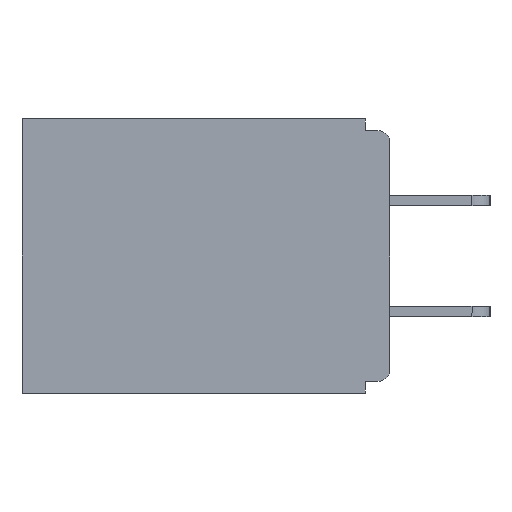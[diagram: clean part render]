
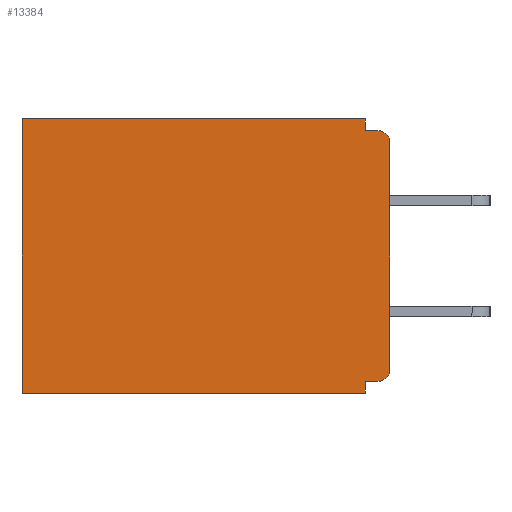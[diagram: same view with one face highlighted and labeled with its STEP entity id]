
A CAD part, left-side view. The second image highlights one B-rep face of the part: STEP entity #13384.
In plain terms, the highlighted planar face has unit normal (-1, 0, 0).
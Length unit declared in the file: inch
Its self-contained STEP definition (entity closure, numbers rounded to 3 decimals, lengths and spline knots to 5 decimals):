
#208 = DIRECTION ( 'NONE',  ( 0., 1., 0. ) ) ;
#1018 = DIRECTION ( 'NONE',  ( 0., 0., -1. ) ) ;
#1232 = CARTESIAN_POINT ( 'NONE',  ( 0.298, 0., -0.015 ) ) ;
#1733 = VECTOR ( 'NONE', #10313, 39.37008 ) ;
#1780 = ORIENTED_EDGE ( 'NONE', *, *, #7760, .T. ) ;
#2868 = EDGE_CURVE ( 'NONE', #8857, #16512, #18832, .T. ) ;
#3001 = ORIENTED_EDGE ( 'NONE', *, *, #2868, .F. ) ;
#3251 = ORIENTED_EDGE ( 'NONE', *, *, #22181, .T. ) ;
#3342 = DIRECTION ( 'NONE',  ( 0., 0., -1. ) ) ;
#3400 = EDGE_CURVE ( 'NONE', #14021, #8857, #15258, .T. ) ;
#3413 = CARTESIAN_POINT ( 'NONE',  ( 0.298, 0.015, -0.015 ) ) ;
#3525 = VECTOR ( 'NONE', #6233, 39.37008 ) ;
#3617 = ORIENTED_EDGE ( 'NONE', *, *, #11317, .F. ) ;
#3928 = EDGE_LOOP ( 'NONE', ( #3251, #20395, #15537, #11468, #1780, #3617, #3001, #13263, #16949, #18435 ) ) ;
#4013 = VERTEX_POINT ( 'NONE', #3413 ) ;
#4075 = DIRECTION ( 'NONE',  ( 0., 0., -1. ) ) ;
#4299 = AXIS2_PLACEMENT_3D ( 'NONE', #11005, #13020, #3342 ) ;
#4337 = EDGE_CURVE ( 'NONE', #23178, #23728, #9349, .T. ) ;
#4567 = EDGE_CURVE ( 'NONE', #14021, #17138, #11123, .T. ) ;
#4752 = FACE_OUTER_BOUND ( 'NONE', #3928, .T. ) ;
#5215 = DIRECTION ( 'NONE',  ( 0., -1., 0. ) ) ;
#5217 = CARTESIAN_POINT ( 'NONE',  ( 0.298, 0., -0.313 ) ) ;
#5281 = DIRECTION ( 'NONE',  ( 0., 0., -1. ) ) ;
#5298 = VECTOR ( 'NONE', #5281, 39.37008 ) ;
#5669 = CARTESIAN_POINT ( 'NONE',  ( 0.298, 0., -0.343 ) ) ;
#6160 = CARTESIAN_POINT ( 'NONE',  ( 0.298, 0.46, -0.343 ) ) ;
#6233 = DIRECTION ( 'NONE',  ( 0., 0., -1. ) ) ;
#6767 = LINE ( 'NONE', #22527, #5298 ) ;
#6958 = VECTOR ( 'NONE', #13476, 39.37008 ) ;
#7760 = EDGE_CURVE ( 'NONE', #23728, #24409, #6767, .T. ) ;
#8609 = CARTESIAN_POINT ( 'NONE',  ( 0.298, 0.46, 0. ) ) ;
#8857 = VERTEX_POINT ( 'NONE', #24695 ) ;
#9024 = LINE ( 'NONE', #20886, #12075 ) ;
#9349 = LINE ( 'NONE', #19607, #14158 ) ;
#9690 = CARTESIAN_POINT ( 'NONE',  ( 0.298, 0., 0. ) ) ;
#10313 = DIRECTION ( 'NONE',  ( 0., 1., 0. ) ) ;
#10436 = AXIS2_PLACEMENT_3D ( 'NONE', #10706, #18234, #1018 ) ;
#10706 = CARTESIAN_POINT ( 'NONE',  ( 0.298, 0.015, -0.313 ) ) ;
#10724 = LINE ( 'NONE', #9690, #24216 ) ;
#11005 = CARTESIAN_POINT ( 'NONE',  ( 0.298, 0., 0. ) ) ;
#11123 = CIRCLE ( 'NONE', #10436, 0.015 ) ;
#11317 = EDGE_CURVE ( 'NONE', #16512, #24409, #21636, .T. ) ;
#11468 = ORIENTED_EDGE ( 'NONE', *, *, #4337, .T. ) ;
#11710 = VERTEX_POINT ( 'NONE', #21645 ) ;
#11959 = EDGE_CURVE ( 'NONE', #23178, #17502, #9024, .T. ) ;
#12075 = VECTOR ( 'NONE', #13386, 39.37008 ) ;
#12385 = LINE ( 'NONE', #1232, #14745 ) ;
#12413 = CARTESIAN_POINT ( 'NONE',  ( 0.298, 0.031, 0. ) ) ;
#13020 = DIRECTION ( 'NONE',  ( 1., 0., 0. ) ) ;
#13126 = CARTESIAN_POINT ( 'NONE',  ( 0.298, 0.015, -0.328 ) ) ;
#13263 = ORIENTED_EDGE ( 'NONE', *, *, #3400, .F. ) ;
#13384 = ADVANCED_FACE ( 'NONE', ( #4752 ), #22449, .F. ) ;
#13386 = DIRECTION ( 'NONE',  ( 0., 0., -1. ) ) ;
#13476 = DIRECTION ( 'NONE',  ( 0., 1., 0. ) ) ;
#13479 = CARTESIAN_POINT ( 'NONE',  ( 0.298, 0.015, -0.03 ) ) ;
#14021 = VERTEX_POINT ( 'NONE', #13126 ) ;
#14037 = EDGE_CURVE ( 'NONE', #11710, #17138, #10724, .T. ) ;
#14073 = CARTESIAN_POINT ( 'NONE',  ( 0.298, 0., -0.328 ) ) ;
#14158 = VECTOR ( 'NONE', #208, 39.37008 ) ;
#14745 = VECTOR ( 'NONE', #5215, 39.37008 ) ;
#15258 = LINE ( 'NONE', #14073, #1733 ) ;
#15456 = CIRCLE ( 'NONE', #18852, 0.015 ) ;
#15537 = ORIENTED_EDGE ( 'NONE', *, *, #11959, .F. ) ;
#16512 = VERTEX_POINT ( 'NONE', #19632 ) ;
#16949 = ORIENTED_EDGE ( 'NONE', *, *, #4567, .T. ) ;
#17138 = VERTEX_POINT ( 'NONE', #5217 ) ;
#17502 = VERTEX_POINT ( 'NONE', #19630 ) ;
#17711 = CARTESIAN_POINT ( 'NONE',  ( 0.298, 0.031, -0.343 ) ) ;
#18234 = DIRECTION ( 'NONE',  ( -1., 0., 0. ) ) ;
#18435 = ORIENTED_EDGE ( 'NONE', *, *, #14037, .F. ) ;
#18832 = LINE ( 'NONE', #17711, #3525 ) ;
#18852 = AXIS2_PLACEMENT_3D ( 'NONE', #13479, #23007, #4075 ) ;
#19607 = CARTESIAN_POINT ( 'NONE',  ( 0.298, 0., 0. ) ) ;
#19630 = CARTESIAN_POINT ( 'NONE',  ( 0.298, 0.031, -0.015 ) ) ;
#19632 = CARTESIAN_POINT ( 'NONE',  ( 0.298, 0.031, -0.343 ) ) ;
#20395 = ORIENTED_EDGE ( 'NONE', *, *, #22680, .F. ) ;
#20886 = CARTESIAN_POINT ( 'NONE',  ( 0.298, 0.031, -0.343 ) ) ;
#21636 = LINE ( 'NONE', #5669, #6958 ) ;
#21645 = CARTESIAN_POINT ( 'NONE',  ( 0.298, 0., -0.03 ) ) ;
#22181 = EDGE_CURVE ( 'NONE', #11710, #4013, #15456, .T. ) ;
#22449 = PLANE ( 'NONE',  #4299 ) ;
#22527 = CARTESIAN_POINT ( 'NONE',  ( 0.298, 0.46, 0. ) ) ;
#22680 = EDGE_CURVE ( 'NONE', #17502, #4013, #12385, .T. ) ;
#22985 = DIRECTION ( 'NONE',  ( 0., 0., -1. ) ) ;
#23007 = DIRECTION ( 'NONE',  ( -1., 0., 0. ) ) ;
#23178 = VERTEX_POINT ( 'NONE', #12413 ) ;
#23728 = VERTEX_POINT ( 'NONE', #8609 ) ;
#24216 = VECTOR ( 'NONE', #22985, 39.37008 ) ;
#24409 = VERTEX_POINT ( 'NONE', #6160 ) ;
#24695 = CARTESIAN_POINT ( 'NONE',  ( 0.298, 0.031, -0.328 ) ) ;
